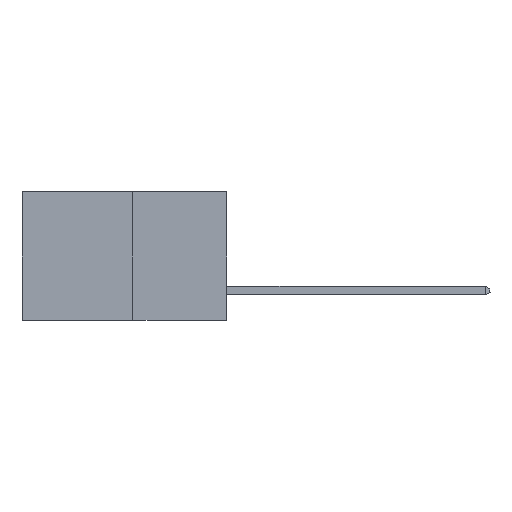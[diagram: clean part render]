
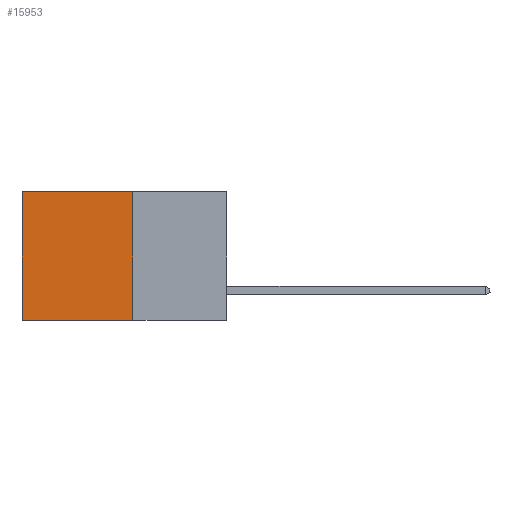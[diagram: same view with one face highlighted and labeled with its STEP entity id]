
A CAD part, left-side view. The second image highlights one B-rep face of the part: STEP entity #15953.
In plain terms, the highlighted planar face has unit normal (-1, 0, 0).
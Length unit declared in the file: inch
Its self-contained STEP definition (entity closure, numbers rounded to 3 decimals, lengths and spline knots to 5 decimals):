
#629 = LINE ( 'NONE', #22226, #15135 ) ;
#731 = ORIENTED_EDGE ( 'NONE', *, *, #8742, .T. ) ;
#1788 = ORIENTED_EDGE ( 'NONE', *, *, #5669, .T. ) ;
#2280 = VERTEX_POINT ( 'NONE', #21672 ) ;
#4691 = DIRECTION ( 'NONE',  ( 0., 0., -1. ) ) ;
#4788 = EDGE_CURVE ( 'NONE', #16435, #2280, #14692, .T. ) ;
#5013 = VECTOR ( 'NONE', #11501, 39.37008 ) ;
#5669 = EDGE_CURVE ( 'NONE', #20973, #2280, #13232, .T. ) ;
#6908 = PLANE ( 'NONE',  #12184 ) ;
#8248 = CARTESIAN_POINT ( 'NONE',  ( 0.277, 0.27, -0.37 ) ) ;
#8405 = VECTOR ( 'NONE', #21124, 39.37008 ) ;
#8622 = CARTESIAN_POINT ( 'NONE',  ( 0.277, 0.27, 0. ) ) ;
#8732 = DIRECTION ( 'NONE',  ( 0., 0., -1. ) ) ;
#8742 = EDGE_CURVE ( 'NONE', #18841, #20973, #629, .T. ) ;
#11501 = DIRECTION ( 'NONE',  ( 0., 1., 0. ) ) ;
#12184 = AXIS2_PLACEMENT_3D ( 'NONE', #19587, #19663, #8732 ) ;
#13077 = CARTESIAN_POINT ( 'NONE',  ( 0.277, 0.27, -0.37 ) ) ;
#13099 = DIRECTION ( 'NONE',  ( 0., 1., 0. ) ) ;
#13232 = LINE ( 'NONE', #21164, #8405 ) ;
#13521 = LINE ( 'NONE', #8248, #22680 ) ;
#13888 = EDGE_CURVE ( 'NONE', #18841, #16435, #13521, .T. ) ;
#14692 = LINE ( 'NONE', #13077, #5013 ) ;
#15135 = VECTOR ( 'NONE', #13099, 39.37008 ) ;
#15188 = ORIENTED_EDGE ( 'NONE', *, *, #13888, .F. ) ;
#15591 = CARTESIAN_POINT ( 'NONE',  ( 0.277, 0.27, -0.37 ) ) ;
#15746 = FACE_OUTER_BOUND ( 'NONE', #20431, .T. ) ;
#15953 = ADVANCED_FACE ( 'NONE', ( #15746 ), #6908, .F. ) ;
#16435 = VERTEX_POINT ( 'NONE', #15591 ) ;
#18841 = VERTEX_POINT ( 'NONE', #8622 ) ;
#19587 = CARTESIAN_POINT ( 'NONE',  ( 0.277, 0.27, -0.37 ) ) ;
#19663 = DIRECTION ( 'NONE',  ( 1., 0., 0. ) ) ;
#20431 = EDGE_LOOP ( 'NONE', ( #1788, #23033, #15188, #731 ) ) ;
#20973 = VERTEX_POINT ( 'NONE', #22701 ) ;
#21124 = DIRECTION ( 'NONE',  ( 0., 0., -1. ) ) ;
#21164 = CARTESIAN_POINT ( 'NONE',  ( 0.277, 0.59, -0.37 ) ) ;
#21672 = CARTESIAN_POINT ( 'NONE',  ( 0.277, 0.59, -0.37 ) ) ;
#22226 = CARTESIAN_POINT ( 'NONE',  ( 0.277, 0.27, 0. ) ) ;
#22680 = VECTOR ( 'NONE', #4691, 39.37008 ) ;
#22701 = CARTESIAN_POINT ( 'NONE',  ( 0.277, 0.59, 0. ) ) ;
#23033 = ORIENTED_EDGE ( 'NONE', *, *, #4788, .F. ) ;
